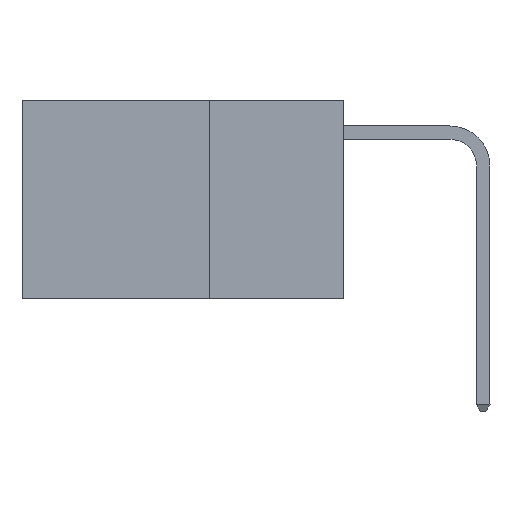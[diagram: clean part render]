
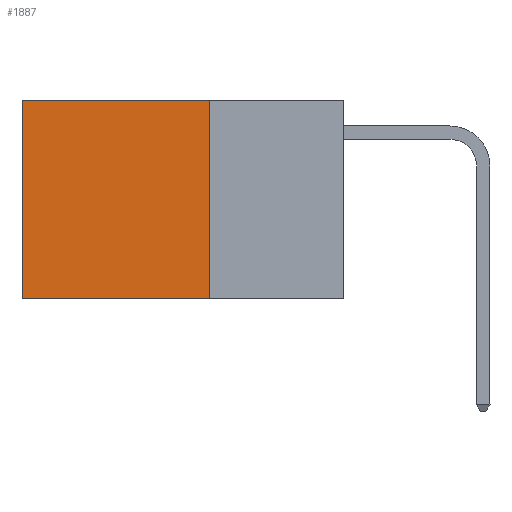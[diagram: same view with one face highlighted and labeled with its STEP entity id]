
A CAD part, left-side view. The second image highlights one B-rep face of the part: STEP entity #1887.
In plain terms, the highlighted planar face has unit normal (-1, 0, 0).
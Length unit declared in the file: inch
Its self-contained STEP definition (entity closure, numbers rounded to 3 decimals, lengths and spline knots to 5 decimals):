
#1351 = CARTESIAN_POINT ( 'NONE',  ( 0.2625, 0.25, 0. ) ) ;
#1887 = ADVANCED_FACE ( 'NONE', ( #2589 ), #6017, .F. ) ;
#2283 = VERTEX_POINT ( 'NONE', #2908 ) ;
#2561 = ORIENTED_EDGE ( 'NONE', *, *, #5053, .F. ) ;
#2589 = FACE_OUTER_BOUND ( 'NONE', #22690, .T. ) ;
#2876 = EDGE_CURVE ( 'NONE', #10010, #17195, #23667, .T. ) ;
#2908 = CARTESIAN_POINT ( 'NONE',  ( 0.2625, 0.6, -0.37 ) ) ;
#3422 = ORIENTED_EDGE ( 'NONE', *, *, #22950, .F. ) ;
#4174 = CARTESIAN_POINT ( 'NONE',  ( 0.2625, 0.25, -0.37 ) ) ;
#4365 = ORIENTED_EDGE ( 'NONE', *, *, #2876, .T. ) ;
#5053 = EDGE_CURVE ( 'NONE', #10010, #16900, #18603, .T. ) ;
#6008 = LINE ( 'NONE', #12808, #21639 ) ;
#6017 = PLANE ( 'NONE',  #13548 ) ;
#7083 = VECTOR ( 'NONE', #16807, 39.37008 ) ;
#7699 = CARTESIAN_POINT ( 'NONE',  ( 0.2625, 0.25, -0.37 ) ) ;
#8046 = LINE ( 'NONE', #7699, #18450 ) ;
#10010 = VERTEX_POINT ( 'NONE', #1351 ) ;
#11283 = DIRECTION ( 'NONE',  ( 1., 0., 0. ) ) ;
#11779 = CARTESIAN_POINT ( 'NONE',  ( 0.2625, 0.25, 0. ) ) ;
#11797 = DIRECTION ( 'NONE',  ( 0., 1., 0. ) ) ;
#12413 = DIRECTION ( 'NONE',  ( 0., 1., 0. ) ) ;
#12808 = CARTESIAN_POINT ( 'NONE',  ( 0.2625, 0.6, 0. ) ) ;
#12915 = DIRECTION ( 'NONE',  ( 0., 0., -1. ) ) ;
#13164 = CARTESIAN_POINT ( 'NONE',  ( 0.2625, 0.6, 0. ) ) ;
#13548 = AXIS2_PLACEMENT_3D ( 'NONE', #11779, #11283, #18881 ) ;
#13627 = EDGE_CURVE ( 'NONE', #17195, #2283, #6008, .T. ) ;
#15347 = ORIENTED_EDGE ( 'NONE', *, *, #13627, .T. ) ;
#16807 = DIRECTION ( 'NONE',  ( 0., 0., -1. ) ) ;
#16900 = VERTEX_POINT ( 'NONE', #4174 ) ;
#16922 = CARTESIAN_POINT ( 'NONE',  ( 0.2625, 0.25, 0. ) ) ;
#17195 = VERTEX_POINT ( 'NONE', #13164 ) ;
#18450 = VECTOR ( 'NONE', #11797, 39.37008 ) ;
#18603 = LINE ( 'NONE', #16922, #7083 ) ;
#18881 = DIRECTION ( 'NONE',  ( 0., 0., -1. ) ) ;
#19927 = VECTOR ( 'NONE', #12413, 39.37008 ) ;
#21639 = VECTOR ( 'NONE', #12915, 39.37008 ) ;
#22690 = EDGE_LOOP ( 'NONE', ( #15347, #3422, #2561, #4365 ) ) ;
#22950 = EDGE_CURVE ( 'NONE', #16900, #2283, #8046, .T. ) ;
#23313 = CARTESIAN_POINT ( 'NONE',  ( 0.2625, 0.25, 0. ) ) ;
#23667 = LINE ( 'NONE', #23313, #19927 ) ;
